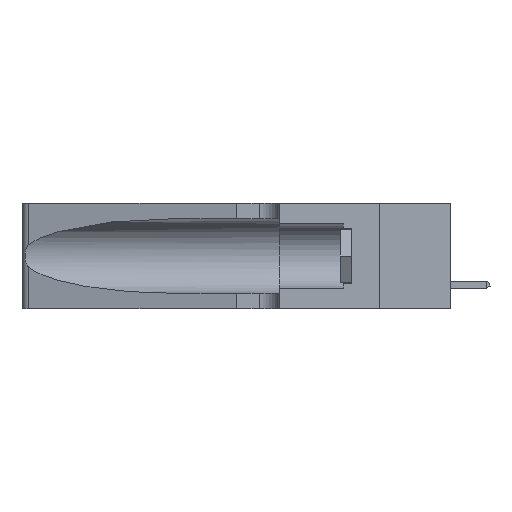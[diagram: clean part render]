
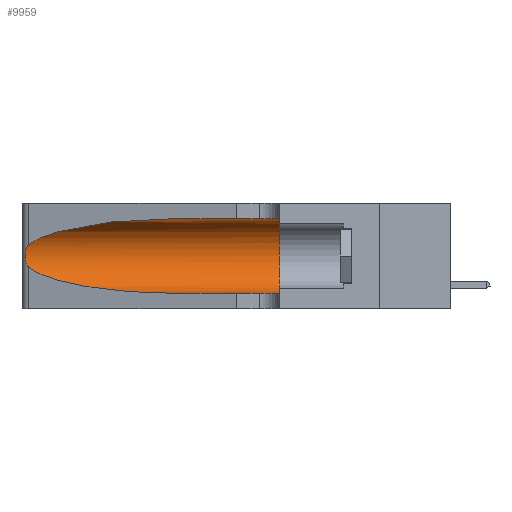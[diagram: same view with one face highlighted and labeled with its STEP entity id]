
A CAD part, left-side view. The second image highlights one B-rep face of the part: STEP entity #9959.
In plain terms, the highlighted cylindrical face has radius 3.308 mm (diameter 6.617 mm), a partial arc.
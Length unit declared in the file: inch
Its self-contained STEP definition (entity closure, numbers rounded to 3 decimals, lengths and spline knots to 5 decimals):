
#585 = VERTEX_POINT ( 'NONE', #7516 ) ;
#1396 = DIRECTION ( 'NONE',  ( 0., 0., 1. ) ) ;
#1819 = CARTESIAN_POINT ( 'NONE',  ( 0.1305, 1.61858, 0.05475 ) ) ;
#2320 = VERTEX_POINT ( 'NONE', #2972 ) ;
#2423 = VECTOR ( 'NONE', #17550, 39.37008 ) ;
#2549 = CARTESIAN_POINT ( 'NONE',  ( 0.18966, 0.96281, 0.05475 ) ) ;
#2713 = EDGE_CURVE ( 'NONE', #10280, #5059, #3525, .T. ) ;
#2972 = CARTESIAN_POINT ( 'NONE',  ( 0.1305, 0.72297, 0.05475 ) ) ;
#3209 = ORIENTED_EDGE ( 'NONE', *, *, #10094, .F. ) ;
#3441 = DIRECTION ( 'NONE',  ( 0., -1., 0. ) ) ;
#3525 =( BOUNDED_CURVE ( )  B_SPLINE_CURVE ( 3, ( #16429, #14901, #10102, #7115 ),
 .UNSPECIFIED., .F., .F. ) 
 B_SPLINE_CURVE_WITH_KNOTS ( ( 4, 4 ),
 ( 1.5708, 2.84003 ),
 .UNSPECIFIED. ) 
 CURVE ( )  GEOMETRIC_REPRESENTATION_ITEM ( )  RATIONAL_B_SPLINE_CURVE ( ( 1., 0.87, 0.87, 1. ) ) 
 REPRESENTATION_ITEM ( '' )  );
#4455 = CARTESIAN_POINT ( 'NONE',  ( 0.1305, 0.35, 0.185 ) ) ;
#4574 = EDGE_LOOP ( 'NONE', ( #17712, #14838, #5011, #11534, #3209, #12183 ) ) ;
#4730 = DIRECTION ( 'NONE',  ( 0., 1., 0. ) ) ;
#4770 =( BOUNDED_CURVE ( )  B_SPLINE_CURVE ( 3, ( #17578, #19528, #2549, #7345 ),
 .UNSPECIFIED., .F., .T. ) 
 B_SPLINE_CURVE_WITH_KNOTS ( ( 4, 4 ),
 ( 3.44316, 4.71239 ),
 .UNSPECIFIED. ) 
 CURVE ( )  GEOMETRIC_REPRESENTATION_ITEM ( )  RATIONAL_B_SPLINE_CURVE ( ( 1., 0.87, 0.87, 1. ) ) 
 REPRESENTATION_ITEM ( '' )  );
#5011 = ORIENTED_EDGE ( 'NONE', *, *, #11825, .T. ) ;
#5059 = VERTEX_POINT ( 'NONE', #7557 ) ;
#5152 = CARTESIAN_POINT ( 'NONE',  ( 0.25487, 1.22718, 0.14631 ) ) ;
#5682 = AXIS2_PLACEMENT_3D ( 'NONE', #4455, #4730, #1396 ) ;
#5738 = CARTESIAN_POINT ( 'NONE',  ( 0.1305, 1.61858, 0.185 ) ) ;
#5774 = EDGE_CURVE ( 'NONE', #2320, #18705, #18018, .T. ) ;
#5872 = CARTESIAN_POINT ( 'NONE',  ( 0.1305, 0.35, 0.05475 ) ) ;
#6166 = DIRECTION ( 'NONE',  ( 0., -1., 0. ) ) ;
#6248 = CARTESIAN_POINT ( 'NONE',  ( 0.25487, 1.22718, 0.14631 ) ) ;
#7115 = CARTESIAN_POINT ( 'NONE',  ( 0.25487, 1.22718, 0.22369 ) ) ;
#7345 = CARTESIAN_POINT ( 'NONE',  ( 0.1305, 0.72297, 0.05475 ) ) ;
#7516 = CARTESIAN_POINT ( 'NONE',  ( 0.1305, 0.35, 0.31525 ) ) ;
#7557 = CARTESIAN_POINT ( 'NONE',  ( 0.25487, 1.22718, 0.22369 ) ) ;
#7838 = CARTESIAN_POINT ( 'NONE',  ( 0.25555, 1.22993, 0.14849 ) ) ;
#8782 = EDGE_CURVE ( 'NONE', #5059, #12511, #14970, .T. ) ;
#9332 = CARTESIAN_POINT ( 'NONE',  ( 0.25787, 1.23484, 0.2124 ) ) ;
#9520 = CARTESIAN_POINT ( 'NONE',  ( 0.1305, 0.72297, 0.31525 ) ) ;
#9669 = CYLINDRICAL_SURFACE ( 'NONE', #15364, 0.13025 ) ;
#9959 = ADVANCED_FACE ( 'NONE', ( #12321 ), #9669, .F. ) ;
#10094 = EDGE_CURVE ( 'NONE', #585, #18705, #16709, .T. ) ;
#10102 = CARTESIAN_POINT ( 'NONE',  ( 0.2373, 1.15595, 0.28018 ) ) ;
#10280 = VERTEX_POINT ( 'NONE', #9520 ) ;
#10598 = CARTESIAN_POINT ( 'NONE',  ( 0.1305, 1.61858, 0.31525 ) ) ;
#10940 = CARTESIAN_POINT ( 'NONE',  ( 0.25789, 1.23486, 0.15765 ) ) ;
#11534 = ORIENTED_EDGE ( 'NONE', *, *, #5774, .T. ) ;
#11825 = EDGE_CURVE ( 'NONE', #12511, #2320, #4770, .T. ) ;
#12183 = ORIENTED_EDGE ( 'NONE', *, *, #14116, .F. ) ;
#12321 = FACE_OUTER_BOUND ( 'NONE', #4574, .T. ) ;
#12500 = CARTESIAN_POINT ( 'NONE',  ( 0.26017, 1.23833, 0.17102 ) ) ;
#12511 = VERTEX_POINT ( 'NONE', #5152 ) ;
#13857 = CARTESIAN_POINT ( 'NONE',  ( 0.26075, 1.23896, 0.178 ) ) ;
#13985 = CARTESIAN_POINT ( 'NONE',  ( 0.25854, 1.2359, 0.20912 ) ) ;
#14116 = EDGE_CURVE ( 'NONE', #10280, #585, #18218, .T. ) ;
#14838 = ORIENTED_EDGE ( 'NONE', *, *, #8782, .T. ) ;
#14901 = CARTESIAN_POINT ( 'NONE',  ( 0.18966, 0.96281, 0.31525 ) ) ;
#14970 = B_SPLINE_CURVE_WITH_KNOTS ( 'NONE', 3,
 ( #17140, #18584, #17071, #9332, #13985, #15499, #17213, #13857, #12500, #18658, #10940, #15401, #7838, #6248 ),
 .UNSPECIFIED., .F., .F.,
 ( 4, 2, 2, 2, 2, 2, 4 ),
 ( 0., 0.00027, 0.00053, 0.00107, 0.0016, 0.00187, 0.00214 ),
 .UNSPECIFIED. ) ;
#15364 = AXIS2_PLACEMENT_3D ( 'NONE', #5738, #6166, #18648 ) ;
#15401 = CARTESIAN_POINT ( 'NONE',  ( 0.25639, 1.23186, 0.15144 ) ) ;
#15499 = CARTESIAN_POINT ( 'NONE',  ( 0.26018, 1.23835, 0.19895 ) ) ;
#16429 = CARTESIAN_POINT ( 'NONE',  ( 0.1305, 0.72297, 0.31525 ) ) ;
#16709 = CIRCLE ( 'NONE', #5682, 0.13025 ) ;
#16738 = VECTOR ( 'NONE', #3441, 39.37008 ) ;
#17071 = CARTESIAN_POINT ( 'NONE',  ( 0.25639, 1.23184, 0.21858 ) ) ;
#17140 = CARTESIAN_POINT ( 'NONE',  ( 0.25487, 1.22718, 0.22369 ) ) ;
#17213 = CARTESIAN_POINT ( 'NONE',  ( 0.26075, 1.23896, 0.19203 ) ) ;
#17550 = DIRECTION ( 'NONE',  ( 0., -1., 0. ) ) ;
#17578 = CARTESIAN_POINT ( 'NONE',  ( 0.25487, 1.22718, 0.14631 ) ) ;
#17712 = ORIENTED_EDGE ( 'NONE', *, *, #2713, .T. ) ;
#18018 = LINE ( 'NONE', #1819, #2423 ) ;
#18218 = LINE ( 'NONE', #10598, #16738 ) ;
#18584 = CARTESIAN_POINT ( 'NONE',  ( 0.25555, 1.22994, 0.2215 ) ) ;
#18648 = DIRECTION ( 'NONE',  ( 0., 0., -1. ) ) ;
#18658 = CARTESIAN_POINT ( 'NONE',  ( 0.25856, 1.23593, 0.16098 ) ) ;
#18705 = VERTEX_POINT ( 'NONE', #5872 ) ;
#19528 = CARTESIAN_POINT ( 'NONE',  ( 0.2373, 1.15595, 0.08982 ) ) ;
